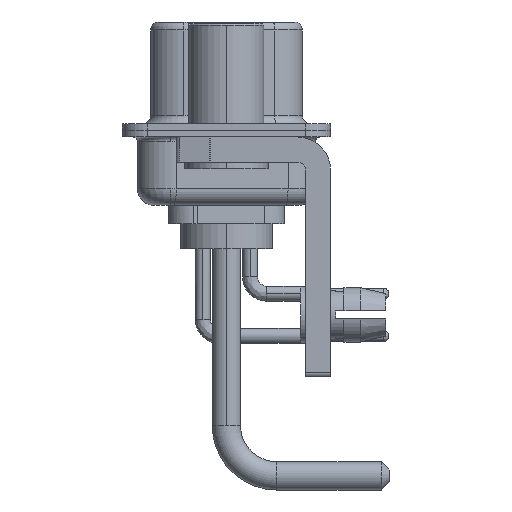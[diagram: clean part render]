
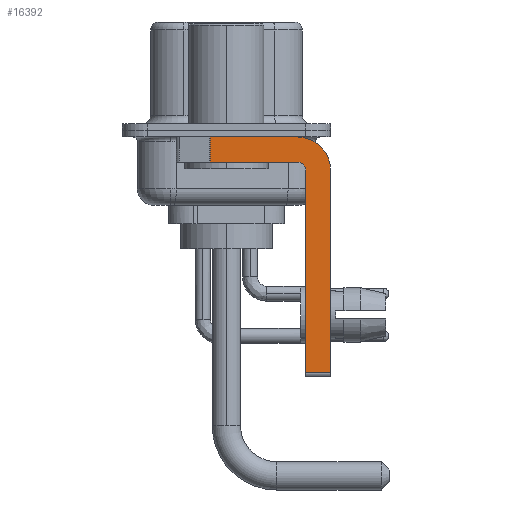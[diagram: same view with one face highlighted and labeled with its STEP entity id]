
A CAD part, left-side view. The second image highlights one B-rep face of the part: STEP entity #16392.
In plain terms, the highlighted planar face has unit normal (-1, 0, 0).
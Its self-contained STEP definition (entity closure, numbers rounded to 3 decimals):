
#296 = CARTESIAN_POINT ( 'NONE',  ( -2.9, -4.25, -1.9 ) ) ;
#928 = CARTESIAN_POINT ( 'NONE',  ( -2.9, 0.978, -0.4 ) ) ;
#938 = CARTESIAN_POINT ( 'NONE',  ( -2.9, -4.75, -14.55 ) ) ;
#2266 = CARTESIAN_POINT ( 'NONE',  ( -2.9, -4.25, -14.55 ) ) ;
#2795 = DIRECTION ( 'NONE',  ( 0., 1., 0. ) ) ;
#3616 = AXIS2_PLACEMENT_3D ( 'NONE', #6483, #8489, #3650 ) ;
#3650 = DIRECTION ( 'NONE',  ( 0., 0., -1. ) ) ;
#4213 = CARTESIAN_POINT ( 'NONE',  ( -2.9, -4.25, -2.4 ) ) ;
#4444 = CARTESIAN_POINT ( 'NONE',  ( -2.9, -4.75, -2.4 ) ) ;
#6107 = DIRECTION ( 'NONE',  ( 1., 0., 0. ) ) ;
#6422 = VERTEX_POINT ( 'NONE', #928 ) ;
#6429 = DIRECTION ( 'NONE',  ( 0., 0., -1. ) ) ;
#6483 = CARTESIAN_POINT ( 'NONE',  ( -2.9, -4.25, -2.4 ) ) ;
#6930 = VECTOR ( 'NONE', #11198, 1000. ) ;
#6940 = DIRECTION ( 'NONE',  ( 0., 0., -1. ) ) ;
#8129 = VERTEX_POINT ( 'NONE', #28946 ) ;
#8212 = ORIENTED_EDGE ( 'NONE', *, *, #15745, .F. ) ;
#8489 = DIRECTION ( 'NONE',  ( 1., 0., 0. ) ) ;
#9082 = VECTOR ( 'NONE', #21372, 1000. ) ;
#9468 = LINE ( 'NONE', #23570, #9082 ) ;
#10508 = CARTESIAN_POINT ( 'NONE',  ( -2.9, -4.25, -2.4 ) ) ;
#10560 = VERTEX_POINT ( 'NONE', #27745 ) ;
#10876 = CARTESIAN_POINT ( 'NONE',  ( -2.9, -4.25, -1.9 ) ) ;
#11013 = VERTEX_POINT ( 'NONE', #4444 ) ;
#11068 = EDGE_CURVE ( 'NONE', #6422, #8129, #25746, .T. ) ;
#11198 = DIRECTION ( 'NONE',  ( 0., -1., 0. ) ) ;
#11730 = ORIENTED_EDGE ( 'NONE', *, *, #27002, .T. ) ;
#11786 = DIRECTION ( 'NONE',  ( 0., -1., 0. ) ) ;
#12810 = VERTEX_POINT ( 'NONE', #938 ) ;
#13586 = VERTEX_POINT ( 'NONE', #15139 ) ;
#13847 = LINE ( 'NONE', #25423, #19947 ) ;
#14598 = EDGE_CURVE ( 'NONE', #8129, #18405, #17091, .T. ) ;
#15055 = CARTESIAN_POINT ( 'NONE',  ( -2.9, -6.25, -2.4 ) ) ;
#15139 = CARTESIAN_POINT ( 'NONE',  ( -2.9, -6.25, -14.55 ) ) ;
#15642 = ORIENTED_EDGE ( 'NONE', *, *, #20233, .T. ) ;
#15745 = EDGE_CURVE ( 'NONE', #25678, #10560, #28770, .T. ) ;
#16344 = CARTESIAN_POINT ( 'NONE',  ( -2.9, -4.75, -14.8 ) ) ;
#16392 = ADVANCED_FACE ( 'NONE', ( #30261 ), #18377, .F. ) ;
#17091 = CIRCLE ( 'NONE', #27044, 2. ) ;
#17747 = DIRECTION ( 'NONE',  ( 0., 0., 1. ) ) ;
#18095 = EDGE_LOOP ( 'NONE', ( #25957, #15642, #8212, #18361, #28819, #11730, #24074, #29482 ) ) ;
#18168 = CIRCLE ( 'NONE', #28641, 0.5 ) ;
#18361 = ORIENTED_EDGE ( 'NONE', *, *, #27363, .F. ) ;
#18377 = PLANE ( 'NONE',  #3616 ) ;
#18405 = VERTEX_POINT ( 'NONE', #15055 ) ;
#19947 = VECTOR ( 'NONE', #6940, 1000. ) ;
#20075 = DIRECTION ( 'NONE',  ( -1., 0., 0. ) ) ;
#20233 = EDGE_CURVE ( 'NONE', #6422, #10560, #9468, .T. ) ;
#21372 = DIRECTION ( 'NONE',  ( 0., 0., -1. ) ) ;
#23234 = LINE ( 'NONE', #16344, #26628 ) ;
#23391 = EDGE_CURVE ( 'NONE', #18405, #13586, #13847, .T. ) ;
#23570 = CARTESIAN_POINT ( 'NONE',  ( -2.9, 0.978, -1.9 ) ) ;
#23694 = CARTESIAN_POINT ( 'NONE',  ( -2.9, 3., -0.4 ) ) ;
#24074 = ORIENTED_EDGE ( 'NONE', *, *, #23391, .F. ) ;
#25132 = VECTOR ( 'NONE', #11786, 1000. ) ;
#25423 = CARTESIAN_POINT ( 'NONE',  ( -2.9, -6.25, -2.4 ) ) ;
#25678 = VERTEX_POINT ( 'NONE', #10876 ) ;
#25746 = LINE ( 'NONE', #23694, #6930 ) ;
#25957 = ORIENTED_EDGE ( 'NONE', *, *, #11068, .F. ) ;
#26021 = LINE ( 'NONE', #2266, #25132 ) ;
#26628 = VECTOR ( 'NONE', #28071, 1000. ) ;
#27002 = EDGE_CURVE ( 'NONE', #12810, #13586, #26021, .T. ) ;
#27003 = EDGE_CURVE ( 'NONE', #12810, #11013, #23234, .T. ) ;
#27044 = AXIS2_PLACEMENT_3D ( 'NONE', #4213, #6107, #6429 ) ;
#27363 = EDGE_CURVE ( 'NONE', #11013, #25678, #18168, .T. ) ;
#27745 = CARTESIAN_POINT ( 'NONE',  ( -2.9, 0.978, -1.9 ) ) ;
#28071 = DIRECTION ( 'NONE',  ( 0., 0., 1. ) ) ;
#28641 = AXIS2_PLACEMENT_3D ( 'NONE', #10508, #20075, #17747 ) ;
#28770 = LINE ( 'NONE', #296, #29068 ) ;
#28819 = ORIENTED_EDGE ( 'NONE', *, *, #27003, .F. ) ;
#28946 = CARTESIAN_POINT ( 'NONE',  ( -2.9, -4.25, -0.4 ) ) ;
#29068 = VECTOR ( 'NONE', #2795, 1000. ) ;
#29482 = ORIENTED_EDGE ( 'NONE', *, *, #14598, .F. ) ;
#30261 = FACE_OUTER_BOUND ( 'NONE', #18095, .T. ) ;
